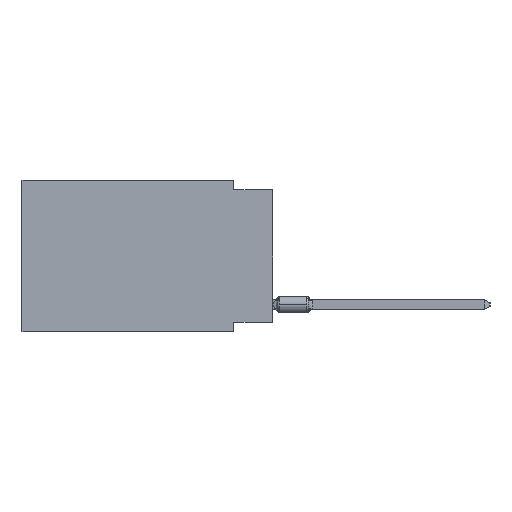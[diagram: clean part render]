
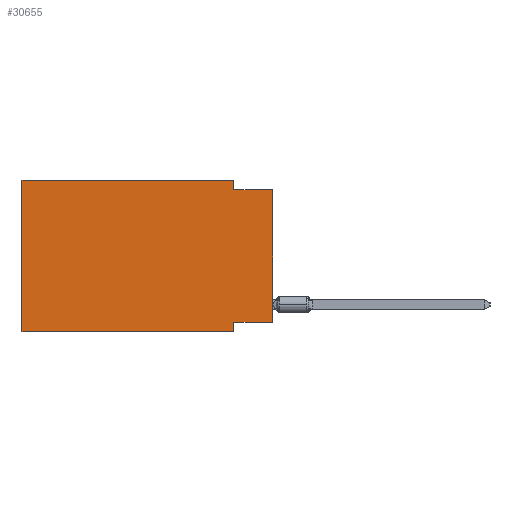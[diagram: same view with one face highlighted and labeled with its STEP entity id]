
A CAD part, left-side view. The second image highlights one B-rep face of the part: STEP entity #30655.
In plain terms, the highlighted planar face has unit normal (-1, 0, 0).
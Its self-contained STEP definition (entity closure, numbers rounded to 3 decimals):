
#661 = CARTESIAN_POINT ( 'NONE',  ( 0., 0., -0.635 ) ) ;
#1181 = VECTOR ( 'NONE', #42069, 1000. ) ;
#2806 = VECTOR ( 'NONE', #11153, 1000. ) ;
#4187 = CARTESIAN_POINT ( 'NONE',  ( 0., 2.54, -0.635 ) ) ;
#4339 = EDGE_CURVE ( 'NONE', #6428, #20583, #26675, .T. ) ;
#5459 = CARTESIAN_POINT ( 'NONE',  ( 0., 2.54, -9.906 ) ) ;
#5650 = AXIS2_PLACEMENT_3D ( 'NONE', #26402, #47360, #61835 ) ;
#6428 = VERTEX_POINT ( 'NONE', #39712 ) ;
#6546 = EDGE_CURVE ( 'NONE', #20583, #24448, #37049, .T. ) ;
#7416 = CARTESIAN_POINT ( 'NONE',  ( 0., 16.383, -9.906 ) ) ;
#7707 = VECTOR ( 'NONE', #46736, 1000. ) ;
#9806 = VERTEX_POINT ( 'NONE', #19451 ) ;
#10353 = ORIENTED_EDGE ( 'NONE', *, *, #4339, .F. ) ;
#11153 = DIRECTION ( 'NONE',  ( 0., -1., 0. ) ) ;
#15027 = ORIENTED_EDGE ( 'NONE', *, *, #50234, .F. ) ;
#15064 = LINE ( 'NONE', #60962, #39417 ) ;
#17415 = VECTOR ( 'NONE', #51006, 1000. ) ;
#17703 = CARTESIAN_POINT ( 'NONE',  ( 0., 2.54, 0. ) ) ;
#19451 = CARTESIAN_POINT ( 'NONE',  ( 0., 0., -9.271 ) ) ;
#20054 = ORIENTED_EDGE ( 'NONE', *, *, #47634, .F. ) ;
#20583 = VERTEX_POINT ( 'NONE', #47831 ) ;
#21119 = ORIENTED_EDGE ( 'NONE', *, *, #62647, .T. ) ;
#22133 = PLANE ( 'NONE',  #5650 ) ;
#22628 = VERTEX_POINT ( 'NONE', #47379 ) ;
#24448 = VERTEX_POINT ( 'NONE', #4187 ) ;
#24938 = ORIENTED_EDGE ( 'NONE', *, *, #47952, .F. ) ;
#26402 = CARTESIAN_POINT ( 'NONE',  ( 0., 16.383, 0. ) ) ;
#26675 = LINE ( 'NONE', #62409, #1181 ) ;
#26795 = DIRECTION ( 'NONE',  ( 0., 0., 1. ) ) ;
#30655 = ADVANCED_FACE ( 'NONE', ( #51985 ), #22133, .F. ) ;
#32316 = LINE ( 'NONE', #7416, #7707 ) ;
#33466 = ORIENTED_EDGE ( 'NONE', *, *, #6546, .F. ) ;
#33750 = VERTEX_POINT ( 'NONE', #57149 ) ;
#34395 = EDGE_CURVE ( 'NONE', #9806, #35739, #15064, .T. ) ;
#35030 = CARTESIAN_POINT ( 'NONE',  ( 0., 2.54, -9.906 ) ) ;
#35042 = DIRECTION ( 'NONE',  ( 0., 0., 1. ) ) ;
#35739 = VERTEX_POINT ( 'NONE', #52702 ) ;
#36211 = VECTOR ( 'NONE', #44545, 1000. ) ;
#36224 = CARTESIAN_POINT ( 'NONE',  ( 0., 0., -9.271 ) ) ;
#37049 = LINE ( 'NONE', #17703, #54833 ) ;
#39417 = VECTOR ( 'NONE', #35042, 1000. ) ;
#39712 = CARTESIAN_POINT ( 'NONE',  ( 0., 16.383, 0. ) ) ;
#39945 = LINE ( 'NONE', #35030, #36211 ) ;
#40384 = VECTOR ( 'NONE', #26795, 1000. ) ;
#42069 = DIRECTION ( 'NONE',  ( 0., -1., 0. ) ) ;
#44545 = DIRECTION ( 'NONE',  ( 0., 0., -1. ) ) ;
#45885 = LINE ( 'NONE', #661, #2806 ) ;
#46383 = LINE ( 'NONE', #36224, #17415 ) ;
#46736 = DIRECTION ( 'NONE',  ( 0., -1., 0. ) ) ;
#47360 = DIRECTION ( 'NONE',  ( 1., 0., 0. ) ) ;
#47379 = CARTESIAN_POINT ( 'NONE',  ( 0., 16.383, -9.906 ) ) ;
#47425 = LINE ( 'NONE', #58258, #40384 ) ;
#47634 = EDGE_CURVE ( 'NONE', #33750, #48179, #39945, .T. ) ;
#47831 = CARTESIAN_POINT ( 'NONE',  ( 0., 2.54, 0. ) ) ;
#47952 = EDGE_CURVE ( 'NONE', #22628, #6428, #47425, .T. ) ;
#48161 = EDGE_CURVE ( 'NONE', #9806, #33750, #46383, .T. ) ;
#48179 = VERTEX_POINT ( 'NONE', #5459 ) ;
#49555 = ORIENTED_EDGE ( 'NONE', *, *, #48161, .F. ) ;
#50234 = EDGE_CURVE ( 'NONE', #24448, #35739, #45885, .T. ) ;
#51006 = DIRECTION ( 'NONE',  ( 0., 1., 0. ) ) ;
#51985 = FACE_OUTER_BOUND ( 'NONE', #53027, .T. ) ;
#52702 = CARTESIAN_POINT ( 'NONE',  ( 0., 0., -0.635 ) ) ;
#53027 = EDGE_LOOP ( 'NONE', ( #62294, #15027, #33466, #10353, #24938, #21119, #20054, #49555 ) ) ;
#54833 = VECTOR ( 'NONE', #57714, 1000. ) ;
#57149 = CARTESIAN_POINT ( 'NONE',  ( 0., 2.54, -9.271 ) ) ;
#57714 = DIRECTION ( 'NONE',  ( 0., 0., -1. ) ) ;
#58258 = CARTESIAN_POINT ( 'NONE',  ( 0., 16.383, 0. ) ) ;
#60962 = CARTESIAN_POINT ( 'NONE',  ( 0., 0., 0. ) ) ;
#61835 = DIRECTION ( 'NONE',  ( 0., 0., -1. ) ) ;
#62294 = ORIENTED_EDGE ( 'NONE', *, *, #34395, .T. ) ;
#62409 = CARTESIAN_POINT ( 'NONE',  ( 0., 16.383, 0. ) ) ;
#62647 = EDGE_CURVE ( 'NONE', #22628, #48179, #32316, .T. ) ;
